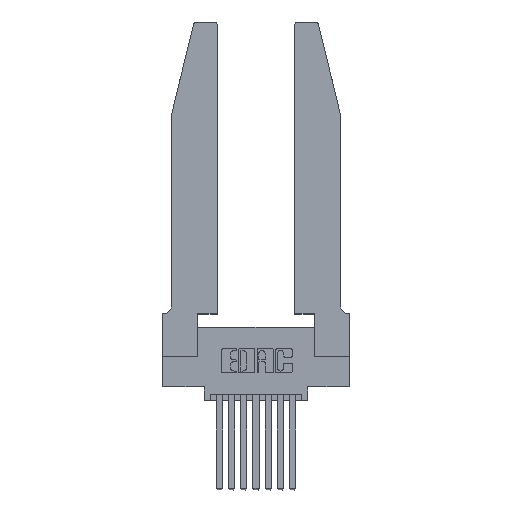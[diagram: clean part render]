
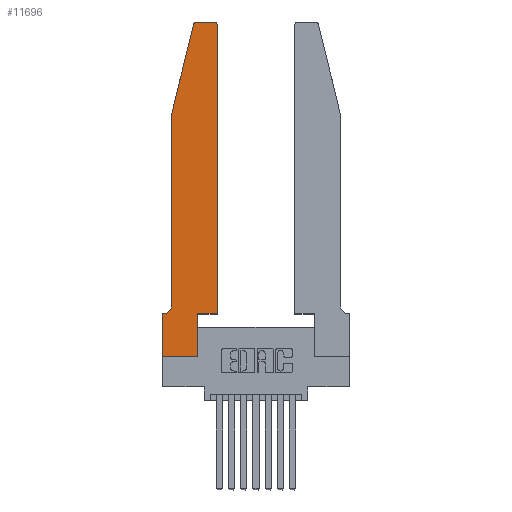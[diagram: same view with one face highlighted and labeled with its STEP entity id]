
A CAD part, top view. The second image highlights one B-rep face of the part: STEP entity #11696.
In plain terms, the highlighted planar face has unit normal (0, 0, 1).
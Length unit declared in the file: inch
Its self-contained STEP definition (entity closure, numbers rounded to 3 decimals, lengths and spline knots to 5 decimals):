
#185 = ORIENTED_EDGE ( 'NONE', *, *, #5873, .T. ) ;
#195 = LINE ( 'NONE', #3271, #12176 ) ;
#457 = ORIENTED_EDGE ( 'NONE', *, *, #9573, .T. ) ;
#478 = AXIS2_PLACEMENT_3D ( 'NONE', #12109, #5344, #13236 ) ;
#725 = ORIENTED_EDGE ( 'NONE', *, *, #5013, .T. ) ;
#1023 = CARTESIAN_POINT ( 'NONE',  ( 0.0755, 2., 0.37 ) ) ;
#1032 = VECTOR ( 'NONE', #9032, 39.37008 ) ;
#1225 = CIRCLE ( 'NONE', #14265, 0.03 ) ;
#1623 = CARTESIAN_POINT ( 'NONE',  ( 0.284, 2.72, 0.37 ) ) ;
#1642 = DIRECTION ( 'NONE',  ( -1., 0., 0. ) ) ;
#1650 = AXIS2_PLACEMENT_3D ( 'NONE', #5285, #13188, #6439 ) ;
#1699 = ORIENTED_EDGE ( 'NONE', *, *, #10785, .T. ) ;
#1704 = CARTESIAN_POINT ( 'NONE',  ( 0.0755, 0.35, 0.37 ) ) ;
#1719 = VERTEX_POINT ( 'NONE', #3620 ) ;
#1874 = CARTESIAN_POINT ( 'NONE',  ( 0.4205, 2.75, 0.37 ) ) ;
#1938 = ORIENTED_EDGE ( 'NONE', *, *, #12762, .T. ) ;
#2300 = DIRECTION ( 'NONE',  ( -0.239, -0.971, 0. ) ) ;
#2421 = VECTOR ( 'NONE', #1642, 39.37008 ) ;
#2683 = EDGE_CURVE ( 'NONE', #1719, #14258, #5592, .T. ) ;
#2796 = CARTESIAN_POINT ( 'NONE',  ( 0.4505, 0.35, 0.37 ) ) ;
#2855 = DIRECTION ( 'NONE',  ( 1., 0., 0. ) ) ;
#2872 = CARTESIAN_POINT ( 'NONE',  ( 0.2865, 0.35, 0.37 ) ) ;
#2916 = VERTEX_POINT ( 'NONE', #12082 ) ;
#3271 = CARTESIAN_POINT ( 'NONE',  ( 0., 0., 0.37 ) ) ;
#3277 = VERTEX_POINT ( 'NONE', #9712 ) ;
#3319 = EDGE_CURVE ( 'NONE', #13142, #2916, #9859, .T. ) ;
#3620 = CARTESIAN_POINT ( 'NONE',  ( 0.0055, 0.35, 0.37 ) ) ;
#3687 = VECTOR ( 'NONE', #2300, 39.37008 ) ;
#3770 = EDGE_LOOP ( 'NONE', ( #5168, #457, #1938, #8083, #13334, #6969, #185, #10207, #1699, #725, #4015, #11500 ) ) ;
#4015 = ORIENTED_EDGE ( 'NONE', *, *, #11678, .T. ) ;
#4049 = DIRECTION ( 'NONE',  ( 0., 1., 0. ) ) ;
#4170 = DIRECTION ( 'NONE',  ( 0., -1., 0. ) ) ;
#4316 = CARTESIAN_POINT ( 'NONE',  ( 0.25487, 2.72718, 0.37 ) ) ;
#4932 = AXIS2_PLACEMENT_3D ( 'NONE', #6396, #14257, #7545 ) ;
#5013 = EDGE_CURVE ( 'NONE', #3277, #9539, #5834, .T. ) ;
#5122 = VECTOR ( 'NONE', #13258, 39.37008 ) ;
#5168 = ORIENTED_EDGE ( 'NONE', *, *, #3319, .T. ) ;
#5280 = DIRECTION ( 'NONE',  ( 0., 1., 0. ) ) ;
#5285 = CARTESIAN_POINT ( 'NONE',  ( 0.4205, 2.72, 0.37 ) ) ;
#5344 = DIRECTION ( 'NONE',  ( 0., 0., -1. ) ) ;
#5592 = LINE ( 'NONE', #1704, #2421 ) ;
#5732 = VERTEX_POINT ( 'NONE', #7641 ) ;
#5834 = LINE ( 'NONE', #6527, #5122 ) ;
#5873 = EDGE_CURVE ( 'NONE', #14258, #8944, #195, .T. ) ;
#6175 = VERTEX_POINT ( 'NONE', #7221 ) ;
#6341 = CARTESIAN_POINT ( 'NONE',  ( 0.4505, 0.35, 0.37 ) ) ;
#6396 = CARTESIAN_POINT ( 'NONE',  ( 0., 0.35, 0.37 ) ) ;
#6439 = DIRECTION ( 'NONE',  ( 1., 0., 0. ) ) ;
#6527 = CARTESIAN_POINT ( 'NONE',  ( 0.4505, 0.35, 0.37 ) ) ;
#6608 = VECTOR ( 'NONE', #5280, 39.37008 ) ;
#6663 = CARTESIAN_POINT ( 'NONE',  ( 0.2865, 0., 0.37 ) ) ;
#6807 = LINE ( 'NONE', #1023, #3687 ) ;
#6842 = VECTOR ( 'NONE', #9473, 39.37008 ) ;
#6969 = ORIENTED_EDGE ( 'NONE', *, *, #2683, .T. ) ;
#6981 = LINE ( 'NONE', #14631, #1032 ) ;
#7102 = EDGE_CURVE ( 'NONE', #6175, #13142, #13029, .T. ) ;
#7221 = CARTESIAN_POINT ( 'NONE',  ( 0.4505, 2.72, 0.37 ) ) ;
#7545 = DIRECTION ( 'NONE',  ( 1., 0., 0. ) ) ;
#7641 = CARTESIAN_POINT ( 'NONE',  ( 0.0755, 2., 0.37 ) ) ;
#7754 = CARTESIAN_POINT ( 'NONE',  ( 0., 0.35, 0.37 ) ) ;
#8083 = ORIENTED_EDGE ( 'NONE', *, *, #14193, .T. ) ;
#8262 = FACE_OUTER_BOUND ( 'NONE', #3770, .T. ) ;
#8288 = VERTEX_POINT ( 'NONE', #4316 ) ;
#8399 = CIRCLE ( 'NONE', #478, 0.07 ) ;
#8761 = CARTESIAN_POINT ( 'NONE',  ( 0.0755, 2., 0.37 ) ) ;
#8944 = VERTEX_POINT ( 'NONE', #9963 ) ;
#9032 = DIRECTION ( 'NONE',  ( 1., 0., 0. ) ) ;
#9283 = VECTOR ( 'NONE', #4170, 39.37008 ) ;
#9473 = DIRECTION ( 'NONE',  ( -1., 0., 0. ) ) ;
#9506 = CARTESIAN_POINT ( 'NONE',  ( 0.2605, 2.75, 0.37 ) ) ;
#9539 = VERTEX_POINT ( 'NONE', #2796 ) ;
#9573 = EDGE_CURVE ( 'NONE', #2916, #8288, #1225, .T. ) ;
#9622 = LINE ( 'NONE', #2872, #6608 ) ;
#9712 = CARTESIAN_POINT ( 'NONE',  ( 0.2865, 0.35, 0.37 ) ) ;
#9794 = DIRECTION ( 'NONE',  ( 0., 0., 1. ) ) ;
#9859 = LINE ( 'NONE', #9506, #6842 ) ;
#9889 = VERTEX_POINT ( 'NONE', #10315 ) ;
#9963 = CARTESIAN_POINT ( 'NONE',  ( 0., 0., 0.37 ) ) ;
#10207 = ORIENTED_EDGE ( 'NONE', *, *, #13225, .T. ) ;
#10230 = EDGE_CURVE ( 'NONE', #9889, #1719, #8399, .T. ) ;
#10315 = CARTESIAN_POINT ( 'NONE',  ( 0.0755, 0.42, 0.37 ) ) ;
#10785 = EDGE_CURVE ( 'NONE', #12575, #3277, #9622, .T. ) ;
#10897 = VECTOR ( 'NONE', #4049, 39.37008 ) ;
#11285 = DIRECTION ( 'NONE',  ( 0., -1., 0. ) ) ;
#11500 = ORIENTED_EDGE ( 'NONE', *, *, #7102, .T. ) ;
#11678 = EDGE_CURVE ( 'NONE', #9539, #6175, #13852, .T. ) ;
#11696 = ADVANCED_FACE ( 'NONE', ( #8262 ), #13147, .T. ) ;
#12082 = CARTESIAN_POINT ( 'NONE',  ( 0.284, 2.75, 0.37 ) ) ;
#12109 = CARTESIAN_POINT ( 'NONE',  ( 0.0055, 0.42, 0.37 ) ) ;
#12176 = VECTOR ( 'NONE', #11285, 39.37008 ) ;
#12240 = LINE ( 'NONE', #8761, #9283 ) ;
#12575 = VERTEX_POINT ( 'NONE', #6663 ) ;
#12762 = EDGE_CURVE ( 'NONE', #8288, #5732, #6807, .T. ) ;
#13029 = CIRCLE ( 'NONE', #1650, 0.03 ) ;
#13142 = VERTEX_POINT ( 'NONE', #1874 ) ;
#13147 = PLANE ( 'NONE',  #4932 ) ;
#13188 = DIRECTION ( 'NONE',  ( 0., 0., 1. ) ) ;
#13225 = EDGE_CURVE ( 'NONE', #8944, #12575, #6981, .T. ) ;
#13236 = DIRECTION ( 'NONE',  ( -1., 0., 0. ) ) ;
#13258 = DIRECTION ( 'NONE',  ( 1., 0., 0. ) ) ;
#13334 = ORIENTED_EDGE ( 'NONE', *, *, #10230, .T. ) ;
#13852 = LINE ( 'NONE', #6341, #10897 ) ;
#14193 = EDGE_CURVE ( 'NONE', #5732, #9889, #12240, .T. ) ;
#14257 = DIRECTION ( 'NONE',  ( 0., 0., 1. ) ) ;
#14258 = VERTEX_POINT ( 'NONE', #7754 ) ;
#14265 = AXIS2_PLACEMENT_3D ( 'NONE', #1623, #9794, #2855 ) ;
#14631 = CARTESIAN_POINT ( 'NONE',  ( 0., 0., 0.37 ) ) ;
